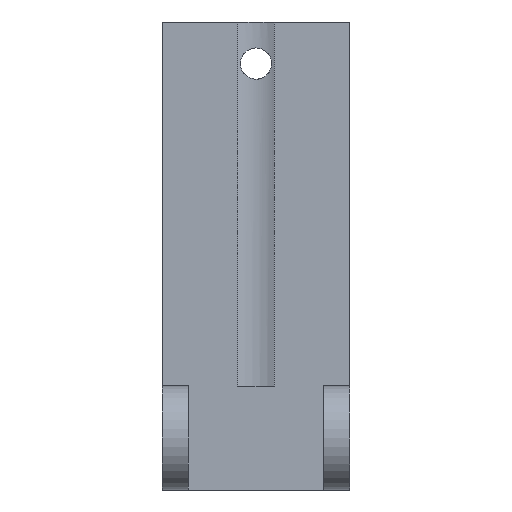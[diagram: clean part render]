
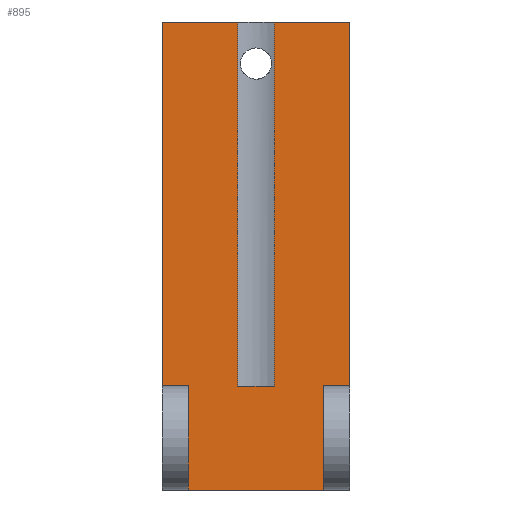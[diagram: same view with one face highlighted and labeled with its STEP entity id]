
A CAD part, front view. The second image highlights one B-rep face of the part: STEP entity #895.
In plain terms, the highlighted planar face has unit normal (0, -1, 0).
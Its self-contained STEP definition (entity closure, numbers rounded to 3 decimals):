
#2 = CARTESIAN_POINT ( 'NONE',  ( -9., -7.5, 40. ) ) ;
#3 = VERTEX_POINT ( 'NONE', #117 ) ;
#7 = EDGE_CURVE ( 'NONE', #1169, #779, #685, .T. ) ;
#11 = EDGE_CURVE ( 'NONE', #1169, #3, #1252, .T. ) ;
#17 = EDGE_CURVE ( 'NONE', #869, #3, #1006, .T. ) ;
#26 = EDGE_CURVE ( 'NONE', #869, #845, #810, .T. ) ;
#32 = EDGE_CURVE ( 'NONE', #854, #845, #789, .T. ) ;
#35 = VECTOR ( 'NONE', #1172, 1000. ) ;
#36 = EDGE_CURVE ( 'NONE', #134, #854, #1611, .T. ) ;
#40 = EDGE_CURVE ( 'NONE', #768, #779, #1320, .T. ) ;
#41 = EDGE_CURVE ( 'NONE', #1426, #134, #157, .T. ) ;
#86 = CARTESIAN_POINT ( 'NONE',  ( 6.5, -7.5, -5. ) ) ;
#103 = DIRECTION ( 'NONE',  ( 1., 0., 0. ) ) ;
#117 = CARTESIAN_POINT ( 'NONE',  ( -1.75, -7.5, 40. ) ) ;
#119 = PLANE ( 'NONE',  #1182 ) ;
#133 = CARTESIAN_POINT ( 'NONE',  ( -9., -7.5, 5. ) ) ;
#134 = VERTEX_POINT ( 'NONE', #749 ) ;
#136 = VECTOR ( 'NONE', #1355, 1000. ) ;
#157 = LINE ( 'NONE', #780, #757 ) ;
#198 = CARTESIAN_POINT ( 'NONE',  ( 1.75, -7.5, 5. ) ) ;
#204 = CARTESIAN_POINT ( 'NONE',  ( 6.5, -7.5, 5. ) ) ;
#219 = CARTESIAN_POINT ( 'NONE',  ( 1.75, -7.5, 40. ) ) ;
#240 = VECTOR ( 'NONE', #381, 1000. ) ;
#269 = VECTOR ( 'NONE', #1368, 1000. ) ;
#308 = VECTOR ( 'NONE', #1597, 1000. ) ;
#316 = LINE ( 'NONE', #611, #240 ) ;
#328 = FACE_OUTER_BOUND ( 'NONE', #640, .T. ) ;
#381 = DIRECTION ( 'NONE',  ( 0., 0., 1. ) ) ;
#398 = CARTESIAN_POINT ( 'NONE',  ( -1.75, -7.5, 40. ) ) ;
#411 = DIRECTION ( 'NONE',  ( 1., 0., 0. ) ) ;
#435 = CARTESIAN_POINT ( 'NONE',  ( -6.5, -7.5, 40. ) ) ;
#438 = CARTESIAN_POINT ( 'NONE',  ( 9., -7.5, 5. ) ) ;
#503 = CARTESIAN_POINT ( 'NONE',  ( -9., -7.5, 40. ) ) ;
#525 = CARTESIAN_POINT ( 'NONE',  ( -9., -7.5, 5. ) ) ;
#529 = EDGE_CURVE ( 'NONE', #1426, #656, #316, .T. ) ;
#611 = CARTESIAN_POINT ( 'NONE',  ( 6.5, -7.5, -5. ) ) ;
#625 = DIRECTION ( 'NONE',  ( 0., 0., 1. ) ) ;
#630 = VECTOR ( 'NONE', #103, 1000. ) ;
#640 = EDGE_LOOP ( 'NONE', ( #767, #781, #818, #859, #936, #977, #992, #1045, #1105, #1217, #1273, #1291 ) ) ;
#656 = VERTEX_POINT ( 'NONE', #204 ) ;
#666 = VECTOR ( 'NONE', #1048, 1000. ) ;
#685 = LINE ( 'NONE', #525, #308 ) ;
#686 = CARTESIAN_POINT ( 'NONE',  ( -1.75, -7.5, 5. ) ) ;
#749 = CARTESIAN_POINT ( 'NONE',  ( -6.5, -7.5, -5. ) ) ;
#757 = VECTOR ( 'NONE', #774, 1000. ) ;
#767 = ORIENTED_EDGE ( 'NONE', *, *, #529, .T. ) ;
#768 = VERTEX_POINT ( 'NONE', #219 ) ;
#774 = DIRECTION ( 'NONE',  ( -1., 0., 0. ) ) ;
#775 = VERTEX_POINT ( 'NONE', #438 ) ;
#779 = VERTEX_POINT ( 'NONE', #198 ) ;
#780 = CARTESIAN_POINT ( 'NONE',  ( 9., -7.5, -5. ) ) ;
#781 = ORIENTED_EDGE ( 'NONE', *, *, #1263, .T. ) ;
#789 = LINE ( 'NONE', #1139, #35 ) ;
#794 = CARTESIAN_POINT ( 'NONE',  ( 9., -7.5, 40. ) ) ;
#810 = LINE ( 'NONE', #1152, #269 ) ;
#818 = ORIENTED_EDGE ( 'NONE', *, *, #1458, .F. ) ;
#843 = EDGE_CURVE ( 'NONE', #768, #1256, #1592, .T. ) ;
#845 = VERTEX_POINT ( 'NONE', #133 ) ;
#854 = VERTEX_POINT ( 'NONE', #1122 ) ;
#859 = ORIENTED_EDGE ( 'NONE', *, *, #843, .F. ) ;
#869 = VERTEX_POINT ( 'NONE', #2 ) ;
#895 = ADVANCED_FACE ( 'NONE', ( #328 ), #119, .F. ) ;
#908 = VECTOR ( 'NONE', #1439, 1000. ) ;
#936 = ORIENTED_EDGE ( 'NONE', *, *, #40, .T. ) ;
#977 = ORIENTED_EDGE ( 'NONE', *, *, #7, .F. ) ;
#988 = VECTOR ( 'NONE', #1248, 1000. ) ;
#992 = ORIENTED_EDGE ( 'NONE', *, *, #11, .T. ) ;
#1002 = CARTESIAN_POINT ( 'NONE',  ( -9., -7.5, 40. ) ) ;
#1006 = LINE ( 'NONE', #1401, #136 ) ;
#1020 = VECTOR ( 'NONE', #411, 1000. ) ;
#1045 = ORIENTED_EDGE ( 'NONE', *, *, #17, .F. ) ;
#1048 = DIRECTION ( 'NONE',  ( 0., 0., 1. ) ) ;
#1053 = CARTESIAN_POINT ( 'NONE',  ( 1.75, -7.5, 40. ) ) ;
#1105 = ORIENTED_EDGE ( 'NONE', *, *, #26, .T. ) ;
#1122 = CARTESIAN_POINT ( 'NONE',  ( -6.5, -7.5, 5. ) ) ;
#1139 = CARTESIAN_POINT ( 'NONE',  ( -9., -7.5, 5. ) ) ;
#1152 = CARTESIAN_POINT ( 'NONE',  ( -9., -7.5, 40. ) ) ;
#1169 = VERTEX_POINT ( 'NONE', #686 ) ;
#1172 = DIRECTION ( 'NONE',  ( -1., 0., 0. ) ) ;
#1182 = AXIS2_PLACEMENT_3D ( 'NONE', #503, #1238, #625 ) ;
#1217 = ORIENTED_EDGE ( 'NONE', *, *, #32, .F. ) ;
#1221 = LINE ( 'NONE', #1554, #908 ) ;
#1238 = DIRECTION ( 'NONE',  ( 0., 1., 0. ) ) ;
#1248 = DIRECTION ( 'NONE',  ( 0., 0., -1. ) ) ;
#1252 = LINE ( 'NONE', #398, #1405 ) ;
#1256 = VERTEX_POINT ( 'NONE', #794 ) ;
#1263 = EDGE_CURVE ( 'NONE', #656, #775, #1328, .T. ) ;
#1273 = ORIENTED_EDGE ( 'NONE', *, *, #36, .F. ) ;
#1291 = ORIENTED_EDGE ( 'NONE', *, *, #41, .F. ) ;
#1320 = LINE ( 'NONE', #1053, #988 ) ;
#1328 = LINE ( 'NONE', #1595, #1020 ) ;
#1355 = DIRECTION ( 'NONE',  ( 1., 0., 0. ) ) ;
#1368 = DIRECTION ( 'NONE',  ( 0., 0., -1. ) ) ;
#1401 = CARTESIAN_POINT ( 'NONE',  ( -9., -7.5, 40. ) ) ;
#1405 = VECTOR ( 'NONE', #1520, 1000. ) ;
#1426 = VERTEX_POINT ( 'NONE', #86 ) ;
#1439 = DIRECTION ( 'NONE',  ( 0., 0., -1. ) ) ;
#1458 = EDGE_CURVE ( 'NONE', #1256, #775, #1221, .T. ) ;
#1520 = DIRECTION ( 'NONE',  ( 0., 0., 1. ) ) ;
#1554 = CARTESIAN_POINT ( 'NONE',  ( 9., -7.5, 40. ) ) ;
#1592 = LINE ( 'NONE', #1002, #630 ) ;
#1595 = CARTESIAN_POINT ( 'NONE',  ( 6.5, -7.5, 5. ) ) ;
#1597 = DIRECTION ( 'NONE',  ( 1., 0., 0. ) ) ;
#1611 = LINE ( 'NONE', #435, #666 ) ;
